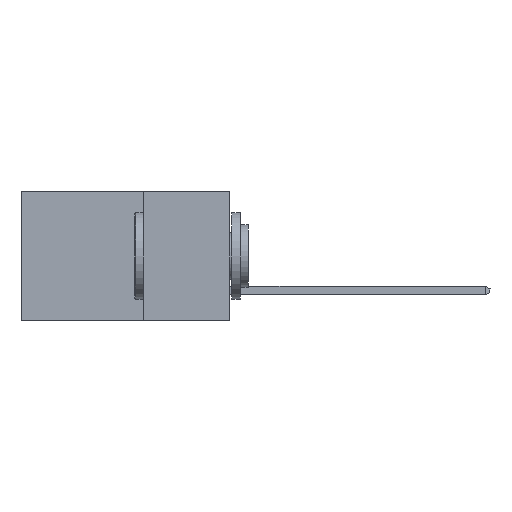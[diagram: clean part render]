
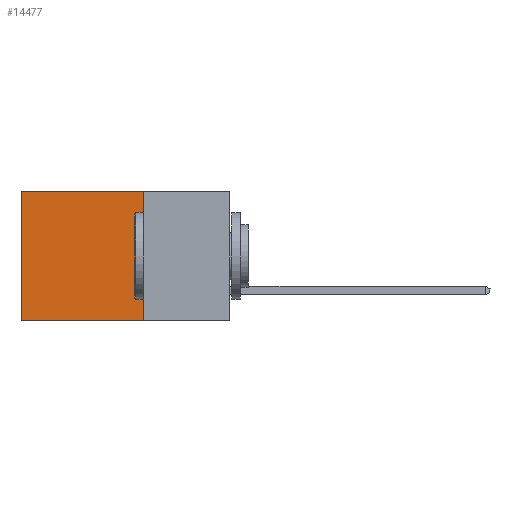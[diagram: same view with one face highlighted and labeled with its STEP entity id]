
A CAD part, left-side view. The second image highlights one B-rep face of the part: STEP entity #14477.
In plain terms, the highlighted planar face has unit normal (-1, 0, 0).
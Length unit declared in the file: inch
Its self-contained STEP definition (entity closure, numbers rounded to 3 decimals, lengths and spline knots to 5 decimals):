
#269 = VECTOR ( 'NONE', #3137, 39.37008 ) ;
#326 = ORIENTED_EDGE ( 'NONE', *, *, #392, .T. ) ;
#368 = CARTESIAN_POINT ( 'NONE',  ( 0.2615, 0.25, 0. ) ) ;
#392 = EDGE_CURVE ( 'NONE', #14743, #6942, #14627, .T. ) ;
#1482 = CARTESIAN_POINT ( 'NONE',  ( 0.2615, 0.6, -0.37 ) ) ;
#1625 = CARTESIAN_POINT ( 'NONE',  ( 0.2615, 0.25, -0.37 ) ) ;
#2593 = EDGE_LOOP ( 'NONE', ( #326, #9438, #12315, #4774 ) ) ;
#2846 = DIRECTION ( 'NONE',  ( 1., 0., 0. ) ) ;
#3094 = VECTOR ( 'NONE', #12172, 39.37008 ) ;
#3137 = DIRECTION ( 'NONE',  ( 0., 1., 0. ) ) ;
#4250 = LINE ( 'NONE', #14901, #269 ) ;
#4774 = ORIENTED_EDGE ( 'NONE', *, *, #10252, .T. ) ;
#5602 = DIRECTION ( 'NONE',  ( 0., 1., 0. ) ) ;
#5804 = EDGE_CURVE ( 'NONE', #10311, #11951, #13561, .T. ) ;
#6036 = CARTESIAN_POINT ( 'NONE',  ( 0.2615, 0.6, -0.37 ) ) ;
#6791 = LINE ( 'NONE', #1625, #12032 ) ;
#6942 = VERTEX_POINT ( 'NONE', #6036 ) ;
#7229 = EDGE_CURVE ( 'NONE', #11951, #6942, #6791, .T. ) ;
#7741 = PLANE ( 'NONE',  #12669 ) ;
#9193 = FACE_OUTER_BOUND ( 'NONE', #2593, .T. ) ;
#9205 = CARTESIAN_POINT ( 'NONE',  ( 0.2615, 0.25, -0.37 ) ) ;
#9362 = DIRECTION ( 'NONE',  ( 0., 0., -1. ) ) ;
#9438 = ORIENTED_EDGE ( 'NONE', *, *, #7229, .F. ) ;
#10252 = EDGE_CURVE ( 'NONE', #10311, #14743, #4250, .T. ) ;
#10311 = VERTEX_POINT ( 'NONE', #368 ) ;
#11951 = VERTEX_POINT ( 'NONE', #9205 ) ;
#12032 = VECTOR ( 'NONE', #5602, 39.37008 ) ;
#12172 = DIRECTION ( 'NONE',  ( 0., 0., -1. ) ) ;
#12315 = ORIENTED_EDGE ( 'NONE', *, *, #5804, .F. ) ;
#12669 = AXIS2_PLACEMENT_3D ( 'NONE', #15737, #2846, #9362 ) ;
#13561 = LINE ( 'NONE', #16148, #3094 ) ;
#13573 = CARTESIAN_POINT ( 'NONE',  ( 0.2615, 0.6, 0. ) ) ;
#13677 = VECTOR ( 'NONE', #15755, 39.37008 ) ;
#14477 = ADVANCED_FACE ( 'NONE', ( #9193 ), #7741, .F. ) ;
#14627 = LINE ( 'NONE', #1482, #13677 ) ;
#14743 = VERTEX_POINT ( 'NONE', #13573 ) ;
#14901 = CARTESIAN_POINT ( 'NONE',  ( 0.2615, 0.25, 0. ) ) ;
#15737 = CARTESIAN_POINT ( 'NONE',  ( 0.2615, 0.25, -0.37 ) ) ;
#15755 = DIRECTION ( 'NONE',  ( 0., 0., -1. ) ) ;
#16148 = CARTESIAN_POINT ( 'NONE',  ( 0.2615, 0.25, -0.37 ) ) ;
